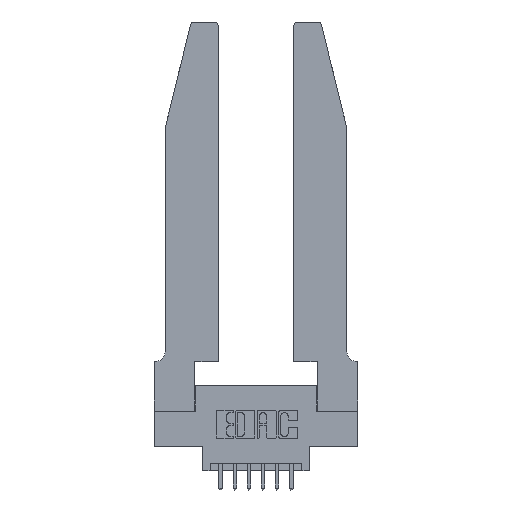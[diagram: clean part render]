
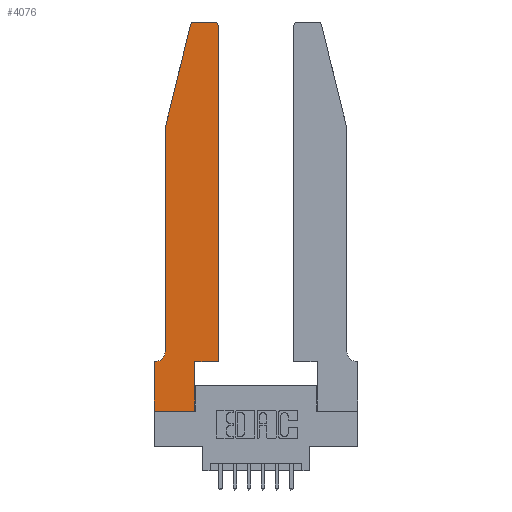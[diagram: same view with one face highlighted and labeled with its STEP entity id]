
A CAD part, top view. The second image highlights one B-rep face of the part: STEP entity #4076.
In plain terms, the highlighted planar face has unit normal (0, 0, 1).
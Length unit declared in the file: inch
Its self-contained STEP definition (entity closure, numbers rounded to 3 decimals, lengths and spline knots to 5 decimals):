
#17 = VERTEX_POINT ( 'NONE', #1079 ) ;
#39 = AXIS2_PLACEMENT_3D ( 'NONE', #841, #1937, #2029 ) ;
#251 = CARTESIAN_POINT ( 'NONE',  ( 0.284, 2.75, 0.37 ) ) ;
#328 = DIRECTION ( 'NONE',  ( 1., 0., 0. ) ) ;
#525 = VECTOR ( 'NONE', #5457, 39.37008 ) ;
#648 = AXIS2_PLACEMENT_3D ( 'NONE', #9247, #8249, #328 ) ;
#655 = ORIENTED_EDGE ( 'NONE', *, *, #9854, .T. ) ;
#819 = VERTEX_POINT ( 'NONE', #5405 ) ;
#841 = CARTESIAN_POINT ( 'NONE',  ( 0.0055, 0.42, 0.37 ) ) ;
#1005 = EDGE_CURVE ( 'NONE', #10997, #17, #5686, .T. ) ;
#1079 = CARTESIAN_POINT ( 'NONE',  ( 0.25487, 2.72718, 0.37 ) ) ;
#1121 = VERTEX_POINT ( 'NONE', #11409 ) ;
#1167 = EDGE_CURVE ( 'NONE', #5923, #3418, #4482, .T. ) ;
#1340 = EDGE_CURVE ( 'NONE', #11784, #7128, #9397, .T. ) ;
#1397 = VERTEX_POINT ( 'NONE', #7693 ) ;
#1465 = VECTOR ( 'NONE', #4907, 39.37008 ) ;
#1601 = ORIENTED_EDGE ( 'NONE', *, *, #9978, .T. ) ;
#1610 = ORIENTED_EDGE ( 'NONE', *, *, #1005, .T. ) ;
#1781 = VECTOR ( 'NONE', #9319, 39.37008 ) ;
#1937 = DIRECTION ( 'NONE',  ( 0., 0., -1. ) ) ;
#2029 = DIRECTION ( 'NONE',  ( -1., 0., 0. ) ) ;
#2245 = DIRECTION ( 'NONE',  ( 0., 0., 1. ) ) ;
#2285 = VERTEX_POINT ( 'NONE', #8135 ) ;
#2403 = PLANE ( 'NONE',  #3971 ) ;
#2610 = DIRECTION ( 'NONE',  ( 1., 0., 0. ) ) ;
#2895 = VERTEX_POINT ( 'NONE', #4775 ) ;
#2944 = ORIENTED_EDGE ( 'NONE', *, *, #6080, .T. ) ;
#3108 = ORIENTED_EDGE ( 'NONE', *, *, #1340, .T. ) ;
#3275 = VECTOR ( 'NONE', #2610, 39.37008 ) ;
#3418 = VERTEX_POINT ( 'NONE', #13084 ) ;
#3466 = EDGE_CURVE ( 'NONE', #9805, #1121, #9504, .T. ) ;
#3490 = CARTESIAN_POINT ( 'NONE',  ( 0.0755, 2., 0.37 ) ) ;
#3803 = ORIENTED_EDGE ( 'NONE', *, *, #4218, .T. ) ;
#3968 = ORIENTED_EDGE ( 'NONE', *, *, #10601, .T. ) ;
#3971 = AXIS2_PLACEMENT_3D ( 'NONE', #10178, #8023, #10221 ) ;
#4051 = LINE ( 'NONE', #3490, #4934 ) ;
#4076 = ADVANCED_FACE ( 'NONE', ( #5076 ), #2403, .T. ) ;
#4218 = EDGE_CURVE ( 'NONE', #3418, #10997, #11888, .T. ) ;
#4268 = LINE ( 'NONE', #11491, #6524 ) ;
#4482 = CIRCLE ( 'NONE', #648, 0.03 ) ;
#4609 = CARTESIAN_POINT ( 'NONE',  ( 0., 0., 0.37 ) ) ;
#4676 = DIRECTION ( 'NONE',  ( 0., -1., 0. ) ) ;
#4775 = CARTESIAN_POINT ( 'NONE',  ( 0.0755, 2., 0.37 ) ) ;
#4907 = DIRECTION ( 'NONE',  ( -0.239, -0.971, 0. ) ) ;
#4934 = VECTOR ( 'NONE', #4676, 39.37008 ) ;
#5076 = FACE_OUTER_BOUND ( 'NONE', #12915, .T. ) ;
#5405 = CARTESIAN_POINT ( 'NONE',  ( 0.0755, 0.42, 0.37 ) ) ;
#5457 = DIRECTION ( 'NONE',  ( 1., 0., 0. ) ) ;
#5686 = CIRCLE ( 'NONE', #8673, 0.03 ) ;
#5733 = DIRECTION ( 'NONE',  ( 1., 0., 0. ) ) ;
#5755 = ORIENTED_EDGE ( 'NONE', *, *, #8868, .T. ) ;
#5923 = VERTEX_POINT ( 'NONE', #12679 ) ;
#6080 = EDGE_CURVE ( 'NONE', #1397, #9805, #10964, .T. ) ;
#6185 = CARTESIAN_POINT ( 'NONE',  ( 0.0055, 0.35, 0.37 ) ) ;
#6408 = CARTESIAN_POINT ( 'NONE',  ( 0.0755, 0.35, 0.37 ) ) ;
#6498 = LINE ( 'NONE', #8050, #1465 ) ;
#6524 = VECTOR ( 'NONE', #8137, 39.37008 ) ;
#6726 = EDGE_CURVE ( 'NONE', #7128, #1397, #12354, .T. ) ;
#6765 = EDGE_CURVE ( 'NONE', #1121, #2285, #10578, .T. ) ;
#6967 = CARTESIAN_POINT ( 'NONE',  ( 0.2605, 2.75, 0.37 ) ) ;
#7128 = VERTEX_POINT ( 'NONE', #13847 ) ;
#7260 = VECTOR ( 'NONE', #7588, 39.37008 ) ;
#7588 = DIRECTION ( 'NONE',  ( -1., 0., 0. ) ) ;
#7693 = CARTESIAN_POINT ( 'NONE',  ( 0., 0., 0.37 ) ) ;
#7750 = CARTESIAN_POINT ( 'NONE',  ( 0.2865, 0.35, 0.37 ) ) ;
#7909 = VECTOR ( 'NONE', #10918, 39.37008 ) ;
#8023 = DIRECTION ( 'NONE',  ( 0., 0., 1. ) ) ;
#8050 = CARTESIAN_POINT ( 'NONE',  ( 0.0755, 2., 0.37 ) ) ;
#8135 = CARTESIAN_POINT ( 'NONE',  ( 0.4505, 0.35, 0.37 ) ) ;
#8137 = DIRECTION ( 'NONE',  ( 0., 1., 0. ) ) ;
#8249 = DIRECTION ( 'NONE',  ( 0., 0., 1. ) ) ;
#8607 = CARTESIAN_POINT ( 'NONE',  ( 0.2865, 0., 0.37 ) ) ;
#8673 = AXIS2_PLACEMENT_3D ( 'NONE', #8967, #2245, #5733 ) ;
#8868 = EDGE_CURVE ( 'NONE', #2285, #5923, #4268, .T. ) ;
#8967 = CARTESIAN_POINT ( 'NONE',  ( 0.284, 2.72, 0.37 ) ) ;
#9068 = VECTOR ( 'NONE', #11630, 39.37008 ) ;
#9247 = CARTESIAN_POINT ( 'NONE',  ( 0.4205, 2.72, 0.37 ) ) ;
#9319 = DIRECTION ( 'NONE',  ( -1., 0., 0. ) ) ;
#9329 = CARTESIAN_POINT ( 'NONE',  ( 0.4505, 0.35, 0.37 ) ) ;
#9397 = LINE ( 'NONE', #6408, #7260 ) ;
#9504 = LINE ( 'NONE', #7750, #7909 ) ;
#9805 = VERTEX_POINT ( 'NONE', #8607 ) ;
#9854 = EDGE_CURVE ( 'NONE', #2895, #819, #4051, .T. ) ;
#9978 = EDGE_CURVE ( 'NONE', #17, #2895, #6498, .T. ) ;
#10167 = CIRCLE ( 'NONE', #39, 0.07 ) ;
#10178 = CARTESIAN_POINT ( 'NONE',  ( 0., 0.35, 0.37 ) ) ;
#10221 = DIRECTION ( 'NONE',  ( 1., 0., 0. ) ) ;
#10578 = LINE ( 'NONE', #9329, #3275 ) ;
#10601 = EDGE_CURVE ( 'NONE', #819, #11784, #10167, .T. ) ;
#10918 = DIRECTION ( 'NONE',  ( 0., 1., 0. ) ) ;
#10964 = LINE ( 'NONE', #14149, #525 ) ;
#10997 = VERTEX_POINT ( 'NONE', #251 ) ;
#11130 = ORIENTED_EDGE ( 'NONE', *, *, #6726, .T. ) ;
#11409 = CARTESIAN_POINT ( 'NONE',  ( 0.2865, 0.35, 0.37 ) ) ;
#11491 = CARTESIAN_POINT ( 'NONE',  ( 0.4505, 0.35, 0.37 ) ) ;
#11630 = DIRECTION ( 'NONE',  ( 0., -1., 0. ) ) ;
#11784 = VERTEX_POINT ( 'NONE', #6185 ) ;
#11888 = LINE ( 'NONE', #6967, #1781 ) ;
#12354 = LINE ( 'NONE', #4609, #9068 ) ;
#12679 = CARTESIAN_POINT ( 'NONE',  ( 0.4505, 2.72, 0.37 ) ) ;
#12915 = EDGE_LOOP ( 'NONE', ( #3803, #1610, #1601, #655, #3968, #3108, #11130, #2944, #13321, #14340, #5755, #14114 ) ) ;
#13084 = CARTESIAN_POINT ( 'NONE',  ( 0.4205, 2.75, 0.37 ) ) ;
#13321 = ORIENTED_EDGE ( 'NONE', *, *, #3466, .T. ) ;
#13847 = CARTESIAN_POINT ( 'NONE',  ( 0., 0.35, 0.37 ) ) ;
#14114 = ORIENTED_EDGE ( 'NONE', *, *, #1167, .T. ) ;
#14149 = CARTESIAN_POINT ( 'NONE',  ( 0., 0., 0.37 ) ) ;
#14340 = ORIENTED_EDGE ( 'NONE', *, *, #6765, .T. ) ;
